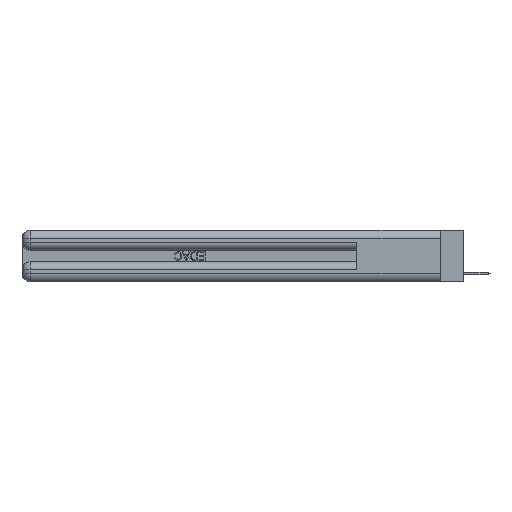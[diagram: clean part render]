
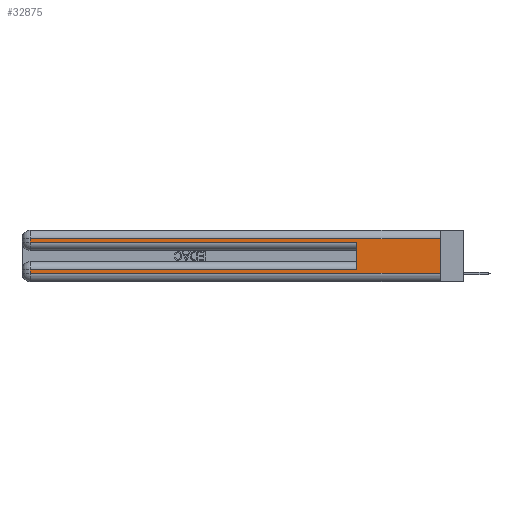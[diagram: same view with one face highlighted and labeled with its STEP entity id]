
A CAD part, left-side view. The second image highlights one B-rep face of the part: STEP entity #32875.
In plain terms, the highlighted planar face has unit normal (-1, 0, 0).
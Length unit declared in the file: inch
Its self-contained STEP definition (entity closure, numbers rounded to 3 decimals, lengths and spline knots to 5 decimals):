
#301 = LINE ( 'NONE', #22126, #11473 ) ;
#726 = PLANE ( 'NONE',  #33192 ) ;
#1963 = LINE ( 'NONE', #10189, #27002 ) ;
#2771 = VERTEX_POINT ( 'NONE', #35210 ) ;
#2804 = CARTESIAN_POINT ( 'NONE',  ( 0., 2.94, 0.31 ) ) ;
#2882 = EDGE_CURVE ( 'NONE', #26003, #2771, #1963, .T. ) ;
#2979 = CARTESIAN_POINT ( 'NONE',  ( 0., 2.94, 0.285 ) ) ;
#4146 = VERTEX_POINT ( 'NONE', #25378 ) ;
#4812 = CARTESIAN_POINT ( 'NONE',  ( 0., 0., 0.37 ) ) ;
#5105 = ORIENTED_EDGE ( 'NONE', *, *, #35005, .T. ) ;
#6215 = VECTOR ( 'NONE', #19500, 39.37008 ) ;
#6292 = VECTOR ( 'NONE', #26625, 39.37008 ) ;
#6809 = LINE ( 'NONE', #28443, #15854 ) ;
#7716 = LINE ( 'NONE', #20973, #10501 ) ;
#8531 = EDGE_CURVE ( 'NONE', #14703, #13273, #34499, .T. ) ;
#8576 = LINE ( 'NONE', #25202, #6215 ) ;
#8637 = ORIENTED_EDGE ( 'NONE', *, *, #30159, .T. ) ;
#9949 = EDGE_CURVE ( 'NONE', #23724, #13273, #34503, .T. ) ;
#10189 = CARTESIAN_POINT ( 'NONE',  ( 0., 0.6, 0.145 ) ) ;
#10501 = VECTOR ( 'NONE', #32391, 39.37008 ) ;
#10526 = VERTEX_POINT ( 'NONE', #2979 ) ;
#11473 = VECTOR ( 'NONE', #33017, 39.37008 ) ;
#13273 = VERTEX_POINT ( 'NONE', #18104 ) ;
#13522 = EDGE_LOOP ( 'NONE', ( #26757, #29060, #23028, #8637, #16433, #33874, #5105, #23146 ) ) ;
#13597 = LINE ( 'NONE', #29857, #32494 ) ;
#14703 = VERTEX_POINT ( 'NONE', #15252 ) ;
#15201 = DIRECTION ( 'NONE',  ( 0., 0., -1. ) ) ;
#15252 = CARTESIAN_POINT ( 'NONE',  ( 0., 0., 0.31 ) ) ;
#15854 = VECTOR ( 'NONE', #23265, 39.37008 ) ;
#16433 = ORIENTED_EDGE ( 'NONE', *, *, #2882, .F. ) ;
#16662 = CARTESIAN_POINT ( 'NONE',  ( 0., 0., 0.37 ) ) ;
#18104 = CARTESIAN_POINT ( 'NONE',  ( 0., 0., 0.06 ) ) ;
#19500 = DIRECTION ( 'NONE',  ( 0., 1., 0. ) ) ;
#19527 = FACE_OUTER_BOUND ( 'NONE', #13522, .T. ) ;
#19869 = DIRECTION ( 'NONE',  ( 0., 0., -1. ) ) ;
#20973 = CARTESIAN_POINT ( 'NONE',  ( 0., 2.94, 0.37 ) ) ;
#22126 = CARTESIAN_POINT ( 'NONE',  ( 0., 2.94, 0.37 ) ) ;
#23028 = ORIENTED_EDGE ( 'NONE', *, *, #24110, .T. ) ;
#23146 = ORIENTED_EDGE ( 'NONE', *, *, #9949, .T. ) ;
#23265 = DIRECTION ( 'NONE',  ( 0., -1., 0. ) ) ;
#23724 = VERTEX_POINT ( 'NONE', #31032 ) ;
#24110 = EDGE_CURVE ( 'NONE', #29065, #10526, #7716, .T. ) ;
#24677 = DIRECTION ( 'NONE',  ( 0., 1., 0. ) ) ;
#25202 = CARTESIAN_POINT ( 'NONE',  ( 0., 0., 0.085 ) ) ;
#25378 = CARTESIAN_POINT ( 'NONE',  ( 0., 2.94, 0.085 ) ) ;
#25733 = VECTOR ( 'NONE', #15201, 39.37008 ) ;
#26003 = VERTEX_POINT ( 'NONE', #29747 ) ;
#26098 = CARTESIAN_POINT ( 'NONE',  ( 0., 0., 0.06 ) ) ;
#26625 = DIRECTION ( 'NONE',  ( 0., -1., 0. ) ) ;
#26757 = ORIENTED_EDGE ( 'NONE', *, *, #8531, .F. ) ;
#27002 = VECTOR ( 'NONE', #32001, 39.37008 ) ;
#28443 = CARTESIAN_POINT ( 'NONE',  ( 0., 0., 0.285 ) ) ;
#29060 = ORIENTED_EDGE ( 'NONE', *, *, #31712, .T. ) ;
#29065 = VERTEX_POINT ( 'NONE', #2804 ) ;
#29747 = CARTESIAN_POINT ( 'NONE',  ( 0., 0.6, 0.085 ) ) ;
#29857 = CARTESIAN_POINT ( 'NONE',  ( 0., 0., 0.31 ) ) ;
#30159 = EDGE_CURVE ( 'NONE', #10526, #2771, #6809, .T. ) ;
#30412 = DIRECTION ( 'NONE',  ( 1., 0., 0. ) ) ;
#31032 = CARTESIAN_POINT ( 'NONE',  ( 0., 2.94, 0.06 ) ) ;
#31712 = EDGE_CURVE ( 'NONE', #14703, #29065, #13597, .T. ) ;
#31868 = EDGE_CURVE ( 'NONE', #26003, #4146, #8576, .T. ) ;
#32001 = DIRECTION ( 'NONE',  ( 0., 0., 1. ) ) ;
#32391 = DIRECTION ( 'NONE',  ( 0., 0., -1. ) ) ;
#32494 = VECTOR ( 'NONE', #24677, 39.37008 ) ;
#32875 = ADVANCED_FACE ( 'NONE', ( #19527 ), #726, .F. ) ;
#33017 = DIRECTION ( 'NONE',  ( 0., 0., -1. ) ) ;
#33192 = AXIS2_PLACEMENT_3D ( 'NONE', #16662, #30412, #19869 ) ;
#33874 = ORIENTED_EDGE ( 'NONE', *, *, #31868, .T. ) ;
#34499 = LINE ( 'NONE', #4812, #25733 ) ;
#34503 = LINE ( 'NONE', #26098, #6292 ) ;
#35005 = EDGE_CURVE ( 'NONE', #4146, #23724, #301, .T. ) ;
#35210 = CARTESIAN_POINT ( 'NONE',  ( 0., 0.6, 0.285 ) ) ;
